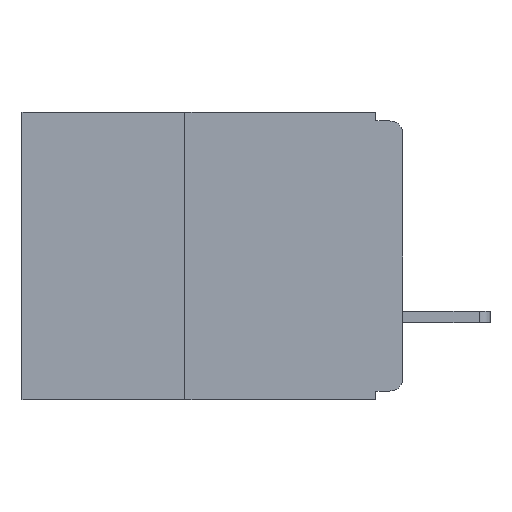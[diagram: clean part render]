
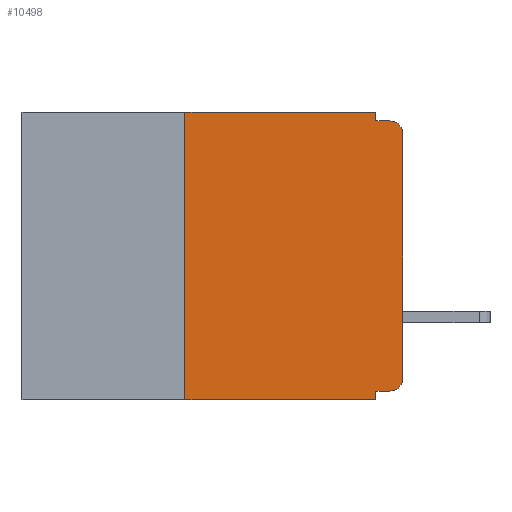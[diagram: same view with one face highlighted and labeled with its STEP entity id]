
A CAD part, left-side view. The second image highlights one B-rep face of the part: STEP entity #10498.
In plain terms, the highlighted planar face has unit normal (-1, 0, 0).
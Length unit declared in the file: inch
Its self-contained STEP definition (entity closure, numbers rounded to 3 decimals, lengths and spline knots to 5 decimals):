
#35 = VERTEX_POINT ( 'NONE', #12349 ) ;
#249 = PLANE ( 'NONE',  #2977 ) ;
#939 = VECTOR ( 'NONE', #25091, 39.37008 ) ;
#1072 = DIRECTION ( 'NONE',  ( 0., 1., 0. ) ) ;
#1173 = EDGE_CURVE ( 'NONE', #19493, #25383, #11257, .T. ) ;
#1952 = ORIENTED_EDGE ( 'NONE', *, *, #23262, .F. ) ;
#1980 = ORIENTED_EDGE ( 'NONE', *, *, #25008, .T. ) ;
#2047 = LINE ( 'NONE', #11529, #12344 ) ;
#2953 = CARTESIAN_POINT ( 'NONE',  ( 0., 0.437, -0.33 ) ) ;
#2977 = AXIS2_PLACEMENT_3D ( 'NONE', #4391, #18769, #6457 ) ;
#3474 = CARTESIAN_POINT ( 'NONE',  ( 0., 0.031, -0.32 ) ) ;
#3823 = CARTESIAN_POINT ( 'NONE',  ( 0., 0., -0.305 ) ) ;
#4391 = CARTESIAN_POINT ( 'NONE',  ( 0., 0.437, 0. ) ) ;
#4511 = EDGE_CURVE ( 'NONE', #9579, #19493, #25239, .T. ) ;
#4617 = VECTOR ( 'NONE', #1072, 39.37008 ) ;
#4618 = VECTOR ( 'NONE', #19446, 39.37008 ) ;
#5048 = CARTESIAN_POINT ( 'NONE',  ( 0., 0.031, -0.33 ) ) ;
#5768 = DIRECTION ( 'NONE',  ( 0., 0., -1. ) ) ;
#6457 = DIRECTION ( 'NONE',  ( 0., 0., -1. ) ) ;
#6828 = CARTESIAN_POINT ( 'NONE',  ( 0., 0.031, -0.33 ) ) ;
#6918 = EDGE_CURVE ( 'NONE', #23250, #17107, #25799, .T. ) ;
#7811 = CARTESIAN_POINT ( 'NONE',  ( 0., 0.015, -0.025 ) ) ;
#7849 = CARTESIAN_POINT ( 'NONE',  ( 0., 0.25, 0. ) ) ;
#8283 = VECTOR ( 'NONE', #19427, 39.37008 ) ;
#9075 = ORIENTED_EDGE ( 'NONE', *, *, #17706, .T. ) ;
#9579 = VERTEX_POINT ( 'NONE', #13434 ) ;
#9901 = DIRECTION ( 'NONE',  ( 0., 0., -1. ) ) ;
#10096 = LINE ( 'NONE', #23649, #4617 ) ;
#10097 = LINE ( 'NONE', #5048, #4618 ) ;
#10436 = ORIENTED_EDGE ( 'NONE', *, *, #6918, .T. ) ;
#10498 = ADVANCED_FACE ( 'NONE', ( #12307 ), #249, .F. ) ;
#10800 = ORIENTED_EDGE ( 'NONE', *, *, #1173, .F. ) ;
#10875 = CIRCLE ( 'NONE', #15391, 0.015 ) ;
#11257 = LINE ( 'NONE', #24999, #939 ) ;
#11529 = CARTESIAN_POINT ( 'NONE',  ( 0., 0., 0. ) ) ;
#11652 = CARTESIAN_POINT ( 'NONE',  ( 0., 0.25, -0.33 ) ) ;
#11786 = CARTESIAN_POINT ( 'NONE',  ( 0., 0.015, -0.305 ) ) ;
#11957 = DIRECTION ( 'NONE',  ( 0., 0., 1. ) ) ;
#12307 = FACE_OUTER_BOUND ( 'NONE', #22864, .T. ) ;
#12344 = VECTOR ( 'NONE', #13599, 39.37008 ) ;
#12349 = CARTESIAN_POINT ( 'NONE',  ( 0., 0., -0.025 ) ) ;
#12711 = CARTESIAN_POINT ( 'NONE',  ( 0., 0.031, -0.01 ) ) ;
#12837 = EDGE_CURVE ( 'NONE', #9579, #23578, #14434, .T. ) ;
#13434 = CARTESIAN_POINT ( 'NONE',  ( 0., 0.25, -0.33 ) ) ;
#13593 = VERTEX_POINT ( 'NONE', #3474 ) ;
#13599 = DIRECTION ( 'NONE',  ( 0., 0., 1. ) ) ;
#13848 = DIRECTION ( 'NONE',  ( 0., 0., -1. ) ) ;
#13964 = CARTESIAN_POINT ( 'NONE',  ( 0., 0.015, -0.32 ) ) ;
#14334 = DIRECTION ( 'NONE',  ( 0., -1., 0. ) ) ;
#14434 = LINE ( 'NONE', #2953, #8283 ) ;
#14680 = ORIENTED_EDGE ( 'NONE', *, *, #12837, .T. ) ;
#14992 = ORIENTED_EDGE ( 'NONE', *, *, #20568, .F. ) ;
#15391 = AXIS2_PLACEMENT_3D ( 'NONE', #7811, #22219, #9901 ) ;
#15654 = ORIENTED_EDGE ( 'NONE', *, *, #4511, .F. ) ;
#16204 = ORIENTED_EDGE ( 'NONE', *, *, #24900, .F. ) ;
#17107 = VERTEX_POINT ( 'NONE', #3823 ) ;
#17157 = CARTESIAN_POINT ( 'NONE',  ( 0., 0.031, 0. ) ) ;
#17179 = EDGE_CURVE ( 'NONE', #22857, #23892, #23126, .T. ) ;
#17706 = EDGE_CURVE ( 'NONE', #35, #23892, #10875, .T. ) ;
#18769 = DIRECTION ( 'NONE',  ( 1., 0., 0. ) ) ;
#19427 = DIRECTION ( 'NONE',  ( 0., -1., 0. ) ) ;
#19446 = DIRECTION ( 'NONE',  ( 0., 0., -1. ) ) ;
#19493 = VERTEX_POINT ( 'NONE', #7849 ) ;
#19842 = LINE ( 'NONE', #22138, #25287 ) ;
#20568 = EDGE_CURVE ( 'NONE', #23250, #13593, #10096, .T. ) ;
#22138 = CARTESIAN_POINT ( 'NONE',  ( 0., 0.031, 0. ) ) ;
#22219 = DIRECTION ( 'NONE',  ( -1., 0., 0. ) ) ;
#22857 = VERTEX_POINT ( 'NONE', #12711 ) ;
#22864 = EDGE_LOOP ( 'NONE', ( #1980, #9075, #26078, #1952, #10800, #15654, #14680, #16204, #14992, #10436 ) ) ;
#23126 = LINE ( 'NONE', #26610, #25021 ) ;
#23250 = VERTEX_POINT ( 'NONE', #13964 ) ;
#23262 = EDGE_CURVE ( 'NONE', #25383, #22857, #19842, .T. ) ;
#23578 = VERTEX_POINT ( 'NONE', #6828 ) ;
#23649 = CARTESIAN_POINT ( 'NONE',  ( 0., 0., -0.32 ) ) ;
#23892 = VERTEX_POINT ( 'NONE', #24251 ) ;
#24251 = CARTESIAN_POINT ( 'NONE',  ( 0., 0.015, -0.01 ) ) ;
#24900 = EDGE_CURVE ( 'NONE', #13593, #23578, #10097, .T. ) ;
#24975 = AXIS2_PLACEMENT_3D ( 'NONE', #11786, #26142, #13848 ) ;
#24999 = CARTESIAN_POINT ( 'NONE',  ( 0., 0.437, 0. ) ) ;
#25008 = EDGE_CURVE ( 'NONE', #17107, #35, #2047, .T. ) ;
#25021 = VECTOR ( 'NONE', #14334, 39.37008 ) ;
#25091 = DIRECTION ( 'NONE',  ( 0., -1., 0. ) ) ;
#25239 = LINE ( 'NONE', #11652, #25890 ) ;
#25287 = VECTOR ( 'NONE', #5768, 39.37008 ) ;
#25383 = VERTEX_POINT ( 'NONE', #17157 ) ;
#25799 = CIRCLE ( 'NONE', #24975, 0.015 ) ;
#25890 = VECTOR ( 'NONE', #11957, 39.37008 ) ;
#26078 = ORIENTED_EDGE ( 'NONE', *, *, #17179, .F. ) ;
#26142 = DIRECTION ( 'NONE',  ( -1., 0., 0. ) ) ;
#26610 = CARTESIAN_POINT ( 'NONE',  ( 0., 0., -0.01 ) ) ;
